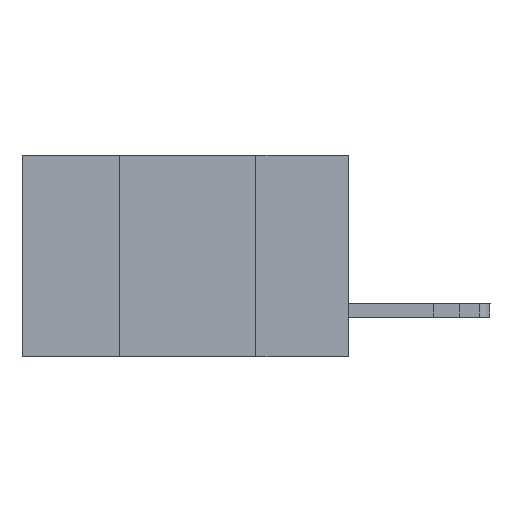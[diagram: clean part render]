
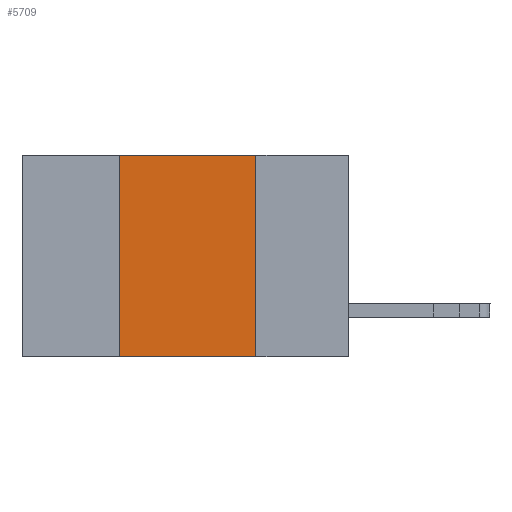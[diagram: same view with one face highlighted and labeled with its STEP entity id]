
A CAD part, left-side view. The second image highlights one B-rep face of the part: STEP entity #5709.
In plain terms, the highlighted planar face has unit normal (-1, 0, 0).
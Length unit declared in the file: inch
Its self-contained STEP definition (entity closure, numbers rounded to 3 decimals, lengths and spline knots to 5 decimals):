
#67 = ORIENTED_EDGE ( 'NONE', *, *, #6896, .F. ) ;
#579 = VERTEX_POINT ( 'NONE', #9020 ) ;
#993 = VECTOR ( 'NONE', #4961, 39.37008 ) ;
#1037 = DIRECTION ( 'NONE',  ( 0., 0., -1. ) ) ;
#1147 = CARTESIAN_POINT ( 'NONE',  ( 0., 0.6, -0.37 ) ) ;
#1524 = VERTEX_POINT ( 'NONE', #11916 ) ;
#2409 = CARTESIAN_POINT ( 'NONE',  ( 0., 0.17, -0.37 ) ) ;
#2425 = PLANE ( 'NONE',  #2607 ) ;
#2572 = CARTESIAN_POINT ( 'NONE',  ( 0., 0.42, 0. ) ) ;
#2607 = AXIS2_PLACEMENT_3D ( 'NONE', #3490, #9204, #1037 ) ;
#2952 = CARTESIAN_POINT ( 'NONE',  ( 0., 0.17, -0.37 ) ) ;
#3403 = LINE ( 'NONE', #1147, #5414 ) ;
#3490 = CARTESIAN_POINT ( 'NONE',  ( 0., 0.6, 0. ) ) ;
#3535 = LINE ( 'NONE', #9479, #993 ) ;
#4051 = LINE ( 'NONE', #2952, #7899 ) ;
#4227 = ORIENTED_EDGE ( 'NONE', *, *, #6931, .F. ) ;
#4359 = LINE ( 'NONE', #14651, #5745 ) ;
#4961 = DIRECTION ( 'NONE',  ( 0., 0., 1. ) ) ;
#5414 = VECTOR ( 'NONE', #12690, 39.37008 ) ;
#5709 = ADVANCED_FACE ( 'NONE', ( #6730 ), #2425, .F. ) ;
#5745 = VECTOR ( 'NONE', #6771, 39.37008 ) ;
#6730 = FACE_OUTER_BOUND ( 'NONE', #10336, .T. ) ;
#6771 = DIRECTION ( 'NONE',  ( 0., -1., 0. ) ) ;
#6896 = EDGE_CURVE ( 'NONE', #1524, #13581, #4051, .T. ) ;
#6931 = EDGE_CURVE ( 'NONE', #10664, #1524, #4359, .T. ) ;
#7705 = EDGE_CURVE ( 'NONE', #579, #10664, #3535, .T. ) ;
#7899 = VECTOR ( 'NONE', #9645, 39.37008 ) ;
#9020 = CARTESIAN_POINT ( 'NONE',  ( 0., 0.42, -0.37 ) ) ;
#9204 = DIRECTION ( 'NONE',  ( 1., 0., 0. ) ) ;
#9479 = CARTESIAN_POINT ( 'NONE',  ( 0., 0.42, -0.37 ) ) ;
#9645 = DIRECTION ( 'NONE',  ( 0., 0., -1. ) ) ;
#10336 = EDGE_LOOP ( 'NONE', ( #67, #4227, #13234, #12806 ) ) ;
#10664 = VERTEX_POINT ( 'NONE', #2572 ) ;
#11916 = CARTESIAN_POINT ( 'NONE',  ( 0., 0.17, 0. ) ) ;
#12690 = DIRECTION ( 'NONE',  ( 0., -1., 0. ) ) ;
#12806 = ORIENTED_EDGE ( 'NONE', *, *, #14619, .T. ) ;
#13234 = ORIENTED_EDGE ( 'NONE', *, *, #7705, .F. ) ;
#13581 = VERTEX_POINT ( 'NONE', #2409 ) ;
#14619 = EDGE_CURVE ( 'NONE', #579, #13581, #3403, .T. ) ;
#14651 = CARTESIAN_POINT ( 'NONE',  ( 0., 0.6, 0. ) ) ;
